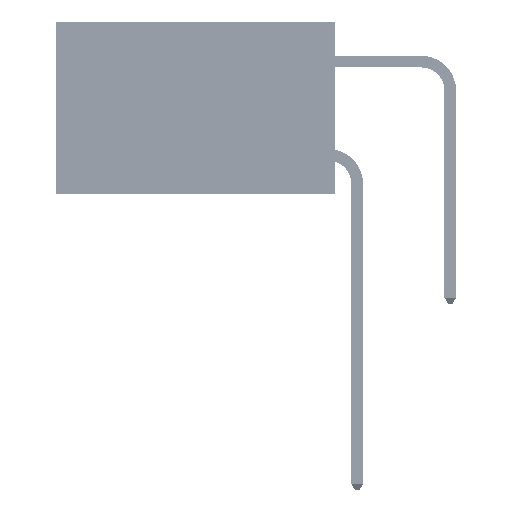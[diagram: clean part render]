
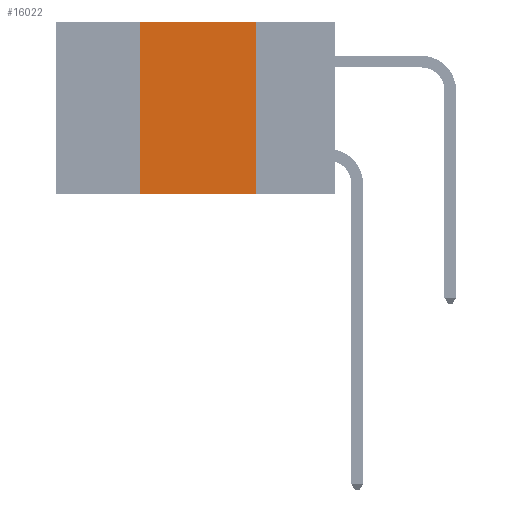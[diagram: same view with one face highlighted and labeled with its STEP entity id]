
A CAD part, left-side view. The second image highlights one B-rep face of the part: STEP entity #16022.
In plain terms, the highlighted planar face has unit normal (-1, 0, 0).
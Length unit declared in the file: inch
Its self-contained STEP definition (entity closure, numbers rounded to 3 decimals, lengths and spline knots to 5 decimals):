
#546 = DIRECTION ( 'NONE',  ( 0., -1., 0. ) ) ;
#674 = PLANE ( 'NONE',  #13333 ) ;
#2345 = VECTOR ( 'NONE', #16399, 39.37008 ) ;
#3876 = CARTESIAN_POINT ( 'NONE',  ( 0., 0.6, 0. ) ) ;
#4632 = CARTESIAN_POINT ( 'NONE',  ( 0., 0.6, 0. ) ) ;
#5416 = LINE ( 'NONE', #19170, #16695 ) ;
#12134 = CARTESIAN_POINT ( 'NONE',  ( 0., 0.17, 0. ) ) ;
#12524 = FACE_OUTER_BOUND ( 'NONE', #17198, .T. ) ;
#13333 = AXIS2_PLACEMENT_3D ( 'NONE', #4632, #15897, #46125 ) ;
#14803 = EDGE_CURVE ( 'NONE', #31392, #44337, #27454, .T. ) ;
#15369 = ORIENTED_EDGE ( 'NONE', *, *, #41617, .F. ) ;
#15897 = DIRECTION ( 'NONE',  ( 1., 0., 0. ) ) ;
#16022 = ADVANCED_FACE ( 'NONE', ( #12524 ), #674, .F. ) ;
#16399 = DIRECTION ( 'NONE',  ( 0., 0., 1. ) ) ;
#16695 = VECTOR ( 'NONE', #45755, 39.37008 ) ;
#17198 = EDGE_LOOP ( 'NONE', ( #44592, #26652, #15369, #26844 ) ) ;
#19170 = CARTESIAN_POINT ( 'NONE',  ( 0., 0.6, -0.37 ) ) ;
#23374 = LINE ( 'NONE', #41287, #46455 ) ;
#26652 = ORIENTED_EDGE ( 'NONE', *, *, #14803, .F. ) ;
#26844 = ORIENTED_EDGE ( 'NONE', *, *, #36498, .T. ) ;
#27377 = VERTEX_POINT ( 'NONE', #29216 ) ;
#27454 = LINE ( 'NONE', #3876, #31002 ) ;
#29216 = CARTESIAN_POINT ( 'NONE',  ( 0., 0.42, -0.37 ) ) ;
#29562 = LINE ( 'NONE', #34877, #2345 ) ;
#30588 = CARTESIAN_POINT ( 'NONE',  ( 0., 0.42, 0. ) ) ;
#31002 = VECTOR ( 'NONE', #546, 39.37008 ) ;
#31392 = VERTEX_POINT ( 'NONE', #30588 ) ;
#32782 = VERTEX_POINT ( 'NONE', #44613 ) ;
#34877 = CARTESIAN_POINT ( 'NONE',  ( 0., 0.42, 0. ) ) ;
#36498 = EDGE_CURVE ( 'NONE', #27377, #32782, #5416, .T. ) ;
#41287 = CARTESIAN_POINT ( 'NONE',  ( 0., 0.17, 0. ) ) ;
#41617 = EDGE_CURVE ( 'NONE', #27377, #31392, #29562, .T. ) ;
#42109 = DIRECTION ( 'NONE',  ( 0., 0., -1. ) ) ;
#44337 = VERTEX_POINT ( 'NONE', #12134 ) ;
#44592 = ORIENTED_EDGE ( 'NONE', *, *, #44913, .F. ) ;
#44613 = CARTESIAN_POINT ( 'NONE',  ( 0., 0.17, -0.37 ) ) ;
#44913 = EDGE_CURVE ( 'NONE', #44337, #32782, #23374, .T. ) ;
#45755 = DIRECTION ( 'NONE',  ( 0., -1., 0. ) ) ;
#46125 = DIRECTION ( 'NONE',  ( 0., 0., -1. ) ) ;
#46455 = VECTOR ( 'NONE', #42109, 39.37008 ) ;
